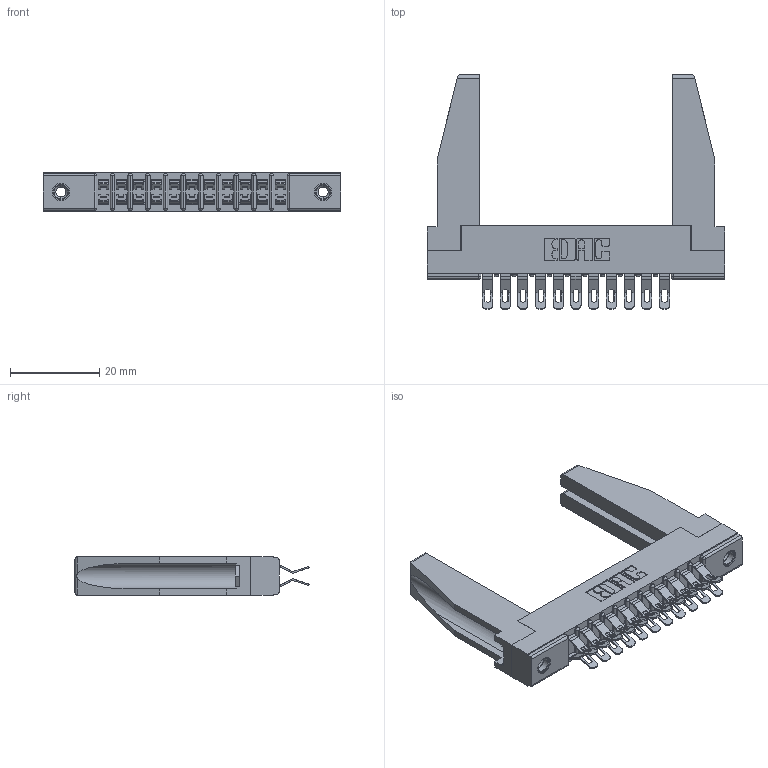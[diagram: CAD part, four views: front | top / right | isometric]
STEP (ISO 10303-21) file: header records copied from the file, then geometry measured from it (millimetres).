
FILE_DESCRIPTION (( 'STEP AP203' ), '1' );
FILE_NAME ('357-022-555-278.STEP', '2019-09-17T21:26:44', ( '' ), ( '' ), 'SwSTEP 2.0', 'SolidWorks 2016', '' );
FILE_SCHEMA (( 'CONFIG_CONTROL_DESIGN' ));
Length unit declared in the file: inch
Products named in the file (5): 307-290-001_555; 307 Part_.156 Dia Mounting Holes; 345-250-001_345-250-001-102; 307-220-078; 357-022-555-278
Assembly tree (27 placements, depth 2):
  357-022-555-278
    307 Part_.156 Dia Mounting Holes
    307-290-001_555  x22
    307-220-078  x2
    345-250-001_345-250-001-102  x2
Bounding box: 66.6 x 52.45 x 8.71 mm (x, y, z)
Volume: 8416.4 mm3; surface area: 11424.6 mm2
Topology: 27 solids, 27 shells, 1602 faces, 4635 edges, 3018 vertices
Faces by surface type: plane 902, cylinder 660, sphere 24, cone 12, torus 4
Entity records: 16580 total; most frequent: CARTESIAN_POINT 2737, ORIENTED_EDGE 2670, DIRECTION 2655, EDGE_CURVE 1335, VECTOR 1003, LINE 1003, VERTEX_POINT 866, AXIS2_PLACEMENT_3D 826
